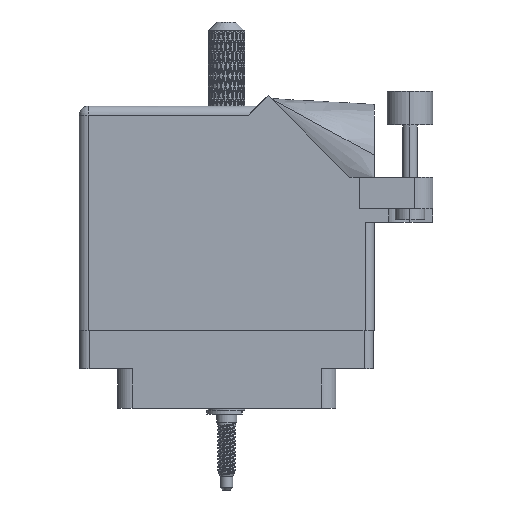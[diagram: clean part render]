
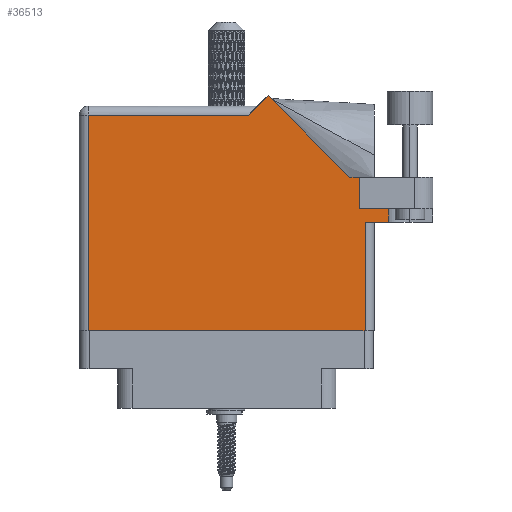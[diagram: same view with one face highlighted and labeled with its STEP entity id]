
A CAD part, front view. The second image highlights one B-rep face of the part: STEP entity #36513.
In plain terms, the highlighted face is planar.
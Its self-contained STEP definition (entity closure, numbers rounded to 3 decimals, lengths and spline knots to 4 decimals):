
#485 = ORIENTED_EDGE ( 'NONE', *, *, #4746, .T. ) ;
#1664 = CARTESIAN_POINT ( 'NONE',  ( 0., 0., 0. ) ) ;
#2360 = AXIS2_PLACEMENT_3D ( 'NONE', #35335, #90984, #100216 ) ;
#3073 = DIRECTION ( 'NONE',  ( -0.707, -0.707, 0. ) ) ;
#3181 = ORIENTED_EDGE ( 'NONE', *, *, #99534, .T. ) ;
#3295 = VECTOR ( 'NONE', #24005, 39.3701 ) ;
#4746 = EDGE_CURVE ( 'NONE', #32329, #95393, #77225, .T. ) ;
#4888 = VECTOR ( 'NONE', #74607, 39.3701 ) ;
#6921 = EDGE_CURVE ( 'NONE', #36986, #79442, #26481, .T. ) ;
#7237 = VERTEX_POINT ( 'NONE', #17156 ) ;
#8165 = EDGE_CURVE ( 'NONE', #95991, #67609, #35103, .T. ) ;
#10455 = DIRECTION ( 'NONE',  ( 1., 0., 0. ) ) ;
#12393 = VECTOR ( 'NONE', #56103, 39.3701 ) ;
#17148 = FACE_OUTER_BOUND ( 'NONE', #19450, .T. ) ;
#17156 = CARTESIAN_POINT ( 'NONE',  ( 1.2877, 1.6007, 0. ) ) ;
#19014 = CARTESIAN_POINT ( 'NONE',  ( 1.91, 1.044, 0. ) ) ;
#19450 = EDGE_LOOP ( 'NONE', ( #51893, #61956, #485, #70694, #52884, #56901, #60324, #60338, #70448, #44783, #3181 ) ) ;
#19612 = VERTEX_POINT ( 'NONE', #77417 ) ;
#21855 = VECTOR ( 'NONE', #62611, 39.3701 ) ;
#23601 = CARTESIAN_POINT ( 'NONE',  ( 0.062, 0., 0. ) ) ;
#24005 = DIRECTION ( 'NONE',  ( -0.707, 0.707, 0. ) ) ;
#24063 = CARTESIAN_POINT ( 'NONE',  ( 2.1115, 0.831, 0. ) ) ;
#24983 = CARTESIAN_POINT ( 'NONE',  ( 0.062, 1.468, 0. ) ) ;
#26298 = LINE ( 'NONE', #51245, #99807 ) ;
#26481 = LINE ( 'NONE', #41734, #4888 ) ;
#27071 = CARTESIAN_POINT ( 'NONE',  ( 1.91, 0.831, 0. ) ) ;
#27190 = PLANE ( 'NONE',  #2360 ) ;
#27224 = CARTESIAN_POINT ( 'NONE',  ( 2.01, 0.737, 0. ) ) ;
#32329 = VERTEX_POINT ( 'NONE', #47720 ) ;
#35103 = LINE ( 'NONE', #72278, #60320 ) ;
#35280 = DIRECTION ( 'NONE',  ( 0., 1., 0. ) ) ;
#35335 = CARTESIAN_POINT ( 'NONE',  ( 0., 1.53, 0. ) ) ;
#36000 = EDGE_CURVE ( 'NONE', #67609, #7237, #45105, .T. ) ;
#36513 = ADVANCED_FACE ( 'NONE', ( #17148 ), #27190, .F. ) ;
#36986 = VERTEX_POINT ( 'NONE', #74512 ) ;
#39728 = EDGE_CURVE ( 'NONE', #19612, #95991, #54965, .T. ) ;
#41734 = CARTESIAN_POINT ( 'NONE',  ( 0., 1.468, 0. ) ) ;
#41811 = LINE ( 'NONE', #43076, #92508 ) ;
#43076 = CARTESIAN_POINT ( 'NONE',  ( 1.948, 0.737, 0. ) ) ;
#44783 = ORIENTED_EDGE ( 'NONE', *, *, #6921, .T. ) ;
#45105 = LINE ( 'NONE', #104798, #3295 ) ;
#47720 = CARTESIAN_POINT ( 'NONE',  ( 1.948, 0.737, 0. ) ) ;
#47948 = CARTESIAN_POINT ( 'NONE',  ( 1.948, 0., 0. ) ) ;
#50400 = LINE ( 'NONE', #23601, #12393 ) ;
#50980 = DIRECTION ( 'NONE',  ( 0., 1., 0. ) ) ;
#51245 = CARTESIAN_POINT ( 'NONE',  ( 1.217, 1.53, 0. ) ) ;
#51893 = ORIENTED_EDGE ( 'NONE', *, *, #61963, .T. ) ;
#51918 = VECTOR ( 'NONE', #76743, 39.3701 ) ;
#52884 = ORIENTED_EDGE ( 'NONE', *, *, #55198, .F. ) ;
#54512 = VERTEX_POINT ( 'NONE', #78272 ) ;
#54965 = LINE ( 'NONE', #27071, #79072 ) ;
#55198 = EDGE_CURVE ( 'NONE', #19612, #104127, #64905, .T. ) ;
#56103 = DIRECTION ( 'NONE',  ( 0., -1., 0. ) ) ;
#56721 = EDGE_CURVE ( 'NONE', #104127, #95393, #84967, .T. ) ;
#56840 = DIRECTION ( 'NONE',  ( 0., -1., 0. ) ) ;
#56850 = EDGE_CURVE ( 'NONE', #101832, #32329, #41811, .T. ) ;
#56901 = ORIENTED_EDGE ( 'NONE', *, *, #39728, .T. ) ;
#57535 = CARTESIAN_POINT ( 'NONE',  ( 2.1115, 1.1618, 0. ) ) ;
#60320 = VECTOR ( 'NONE', #70883, 39.3701 ) ;
#60324 = ORIENTED_EDGE ( 'NONE', *, *, #8165, .T. ) ;
#60338 = ORIENTED_EDGE ( 'NONE', *, *, #36000, .T. ) ;
#61956 = ORIENTED_EDGE ( 'NONE', *, *, #56850, .T. ) ;
#61963 = EDGE_CURVE ( 'NONE', #54512, #101832, #99039, .T. ) ;
#62611 = DIRECTION ( 'NONE',  ( 1., 0., 0. ) ) ;
#64905 = LINE ( 'NONE', #78573, #21855 ) ;
#67208 = VECTOR ( 'NONE', #10455, 39.3701 ) ;
#67609 = VERTEX_POINT ( 'NONE', #85389 ) ;
#70448 = ORIENTED_EDGE ( 'NONE', *, *, #101386, .T. ) ;
#70694 = ORIENTED_EDGE ( 'NONE', *, *, #56721, .F. ) ;
#70883 = DIRECTION ( 'NONE',  ( -1., 0., 0. ) ) ;
#72278 = CARTESIAN_POINT ( 'NONE',  ( 2.41, 1.044, 0. ) ) ;
#73584 = VECTOR ( 'NONE', #56840, 39.3701 ) ;
#74512 = CARTESIAN_POINT ( 'NONE',  ( 1.155, 1.468, 0. ) ) ;
#74607 = DIRECTION ( 'NONE',  ( -1., 0., 0. ) ) ;
#76743 = DIRECTION ( 'NONE',  ( 1., 0., 0. ) ) ;
#77225 = LINE ( 'NONE', #27224, #51918 ) ;
#77417 = CARTESIAN_POINT ( 'NONE',  ( 1.91, 0.831, 0. ) ) ;
#78272 = CARTESIAN_POINT ( 'NONE',  ( 0.062, 0., 0. ) ) ;
#78573 = CARTESIAN_POINT ( 'NONE',  ( 1.91, 0.831, 0. ) ) ;
#79072 = VECTOR ( 'NONE', #50980, 39.3701 ) ;
#79442 = VERTEX_POINT ( 'NONE', #24983 ) ;
#84967 = LINE ( 'NONE', #57535, #73584 ) ;
#85389 = CARTESIAN_POINT ( 'NONE',  ( 1.8444, 1.044, 0. ) ) ;
#90984 = DIRECTION ( 'NONE',  ( 0., 0., -1. ) ) ;
#92508 = VECTOR ( 'NONE', #35280, 39.3701 ) ;
#95393 = VERTEX_POINT ( 'NONE', #104117 ) ;
#95991 = VERTEX_POINT ( 'NONE', #19014 ) ;
#99039 = LINE ( 'NONE', #1664, #67208 ) ;
#99534 = EDGE_CURVE ( 'NONE', #79442, #54512, #50400, .T. ) ;
#99807 = VECTOR ( 'NONE', #3073, 39.3701 ) ;
#100216 = DIRECTION ( 'NONE',  ( -1., 0., 0. ) ) ;
#101386 = EDGE_CURVE ( 'NONE', #7237, #36986, #26298, .T. ) ;
#101832 = VERTEX_POINT ( 'NONE', #47948 ) ;
#104117 = CARTESIAN_POINT ( 'NONE',  ( 2.1115, 0.737, 0. ) ) ;
#104127 = VERTEX_POINT ( 'NONE', #24063 ) ;
#104798 = CARTESIAN_POINT ( 'NONE',  ( 1.8444, 1.044, 0. ) ) ;
